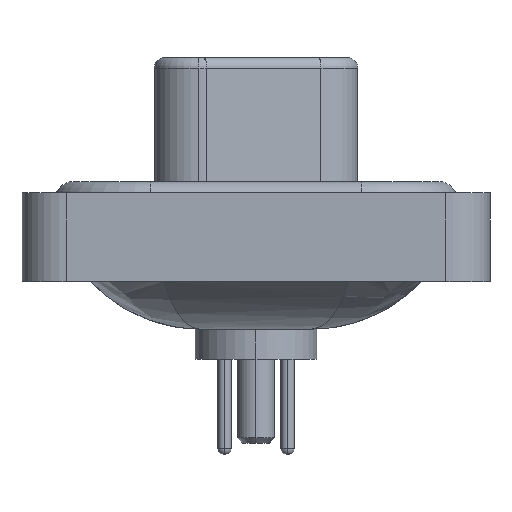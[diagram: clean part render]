
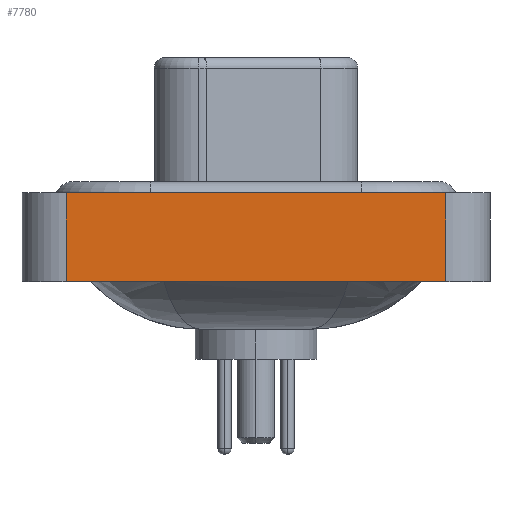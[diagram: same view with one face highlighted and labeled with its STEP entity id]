
A CAD part, left-side view. The second image highlights one B-rep face of the part: STEP entity #7780.
In plain terms, the highlighted planar face has unit normal (-1, 0, 0).
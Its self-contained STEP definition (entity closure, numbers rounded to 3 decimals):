
#607 = LINE ( 'NONE', #10576, #16264 ) ;
#739 = ORIENTED_EDGE ( 'NONE', *, *, #20078, .F. ) ;
#975 = DIRECTION ( 'NONE',  ( -1., 0., 0. ) ) ;
#1172 = PLANE ( 'NONE',  #11920 ) ;
#1337 = EDGE_CURVE ( 'NONE', #3048, #3020, #11521, .T. ) ;
#3020 = VERTEX_POINT ( 'NONE', #6666 ) ;
#3048 = VERTEX_POINT ( 'NONE', #18952 ) ;
#4333 = FACE_OUTER_BOUND ( 'NONE', #14007, .T. ) ;
#4529 = LINE ( 'NONE', #21842, #10020 ) ;
#5287 = EDGE_CURVE ( 'NONE', #7254, #16769, #14059, .T. ) ;
#5322 = DIRECTION ( 'NONE',  ( 0., -1., 0. ) ) ;
#5845 = EDGE_CURVE ( 'NONE', #7254, #3048, #4529, .T. ) ;
#6228 = VECTOR ( 'NONE', #16417, 1000. ) ;
#6666 = CARTESIAN_POINT ( 'NONE',  ( -7.35, -8.55, 0.4 ) ) ;
#7254 = VERTEX_POINT ( 'NONE', #18403 ) ;
#7780 = ADVANCED_FACE ( 'NONE', ( #4333 ), #1172, .T. ) ;
#10020 = VECTOR ( 'NONE', #18280, 1000. ) ;
#10576 = CARTESIAN_POINT ( 'NONE',  ( -7.35, -8.55, 0.4 ) ) ;
#11521 = LINE ( 'NONE', #16890, #19405 ) ;
#11920 = AXIS2_PLACEMENT_3D ( 'NONE', #17878, #975, #14630 ) ;
#14007 = EDGE_LOOP ( 'NONE', ( #15989, #739, #21828, #18629 ) ) ;
#14059 = LINE ( 'NONE', #19567, #6228 ) ;
#14630 = DIRECTION ( 'NONE',  ( 0., 0., 1. ) ) ;
#15989 = ORIENTED_EDGE ( 'NONE', *, *, #1337, .T. ) ;
#16264 = VECTOR ( 'NONE', #5322, 1000. ) ;
#16417 = DIRECTION ( 'NONE',  ( 0., 0., 1. ) ) ;
#16687 = DIRECTION ( 'NONE',  ( 0., 0., 1. ) ) ;
#16769 = VERTEX_POINT ( 'NONE', #21123 ) ;
#16890 = CARTESIAN_POINT ( 'NONE',  ( -7.35, -8.55, -3.6 ) ) ;
#17878 = CARTESIAN_POINT ( 'NONE',  ( -7.35, -8.55, -3.6 ) ) ;
#18280 = DIRECTION ( 'NONE',  ( 0., -1., 0. ) ) ;
#18403 = CARTESIAN_POINT ( 'NONE',  ( -7.35, 8.55, -3.6 ) ) ;
#18629 = ORIENTED_EDGE ( 'NONE', *, *, #5845, .T. ) ;
#18952 = CARTESIAN_POINT ( 'NONE',  ( -7.35, -8.55, -3.6 ) ) ;
#19405 = VECTOR ( 'NONE', #16687, 1000. ) ;
#19567 = CARTESIAN_POINT ( 'NONE',  ( -7.35, 8.55, -3.6 ) ) ;
#20078 = EDGE_CURVE ( 'NONE', #16769, #3020, #607, .T. ) ;
#21123 = CARTESIAN_POINT ( 'NONE',  ( -7.35, 8.55, 0.4 ) ) ;
#21828 = ORIENTED_EDGE ( 'NONE', *, *, #5287, .F. ) ;
#21842 = CARTESIAN_POINT ( 'NONE',  ( -7.35, -8.55, -3.6 ) ) ;
